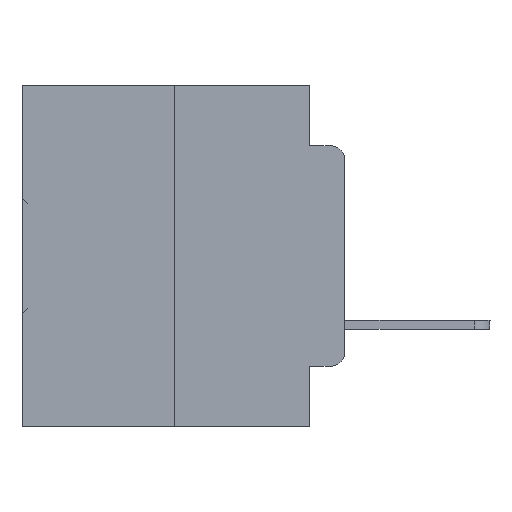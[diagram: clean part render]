
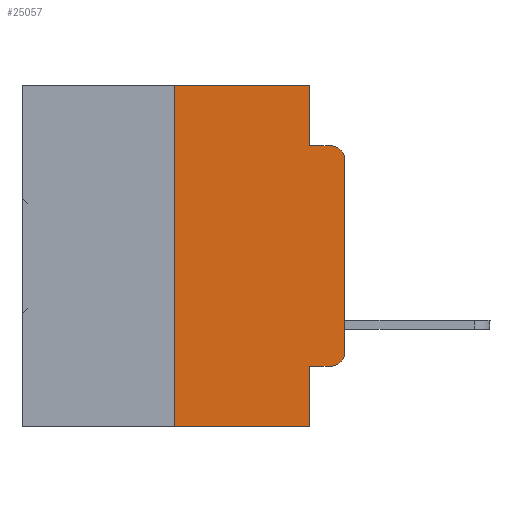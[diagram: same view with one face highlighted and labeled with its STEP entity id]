
A CAD part, left-side view. The second image highlights one B-rep face of the part: STEP entity #25057.
In plain terms, the highlighted planar face has unit normal (-1, 0, 0).
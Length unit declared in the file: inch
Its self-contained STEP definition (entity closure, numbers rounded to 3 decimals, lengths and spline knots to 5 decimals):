
#1318 = CARTESIAN_POINT ( 'NONE',  ( 0., 0.051, 0. ) ) ;
#2047 = LINE ( 'NONE', #31081, #30390 ) ;
#2204 = VECTOR ( 'NONE', #14215, 39.37008 ) ;
#2212 = DIRECTION ( 'NONE',  ( -1., 0., 0. ) ) ;
#2331 = EDGE_CURVE ( 'NONE', #7059, #11870, #3549, .T. ) ;
#2348 = CARTESIAN_POINT ( 'NONE',  ( 0., 0.473, 0. ) ) ;
#2488 = CARTESIAN_POINT ( 'NONE',  ( 0., 0., -0.3915 ) ) ;
#2904 = CARTESIAN_POINT ( 'NONE',  ( 0., 0.25, 0. ) ) ;
#3352 = VECTOR ( 'NONE', #30201, 39.37008 ) ;
#3549 = LINE ( 'NONE', #2904, #31123 ) ;
#3977 = DIRECTION ( 'NONE',  ( 0., 0., -1. ) ) ;
#4874 = DIRECTION ( 'NONE',  ( 0., 0., -1. ) ) ;
#4950 = EDGE_CURVE ( 'NONE', #33336, #5134, #11704, .T. ) ;
#5134 = VERTEX_POINT ( 'NONE', #10693 ) ;
#5249 = CARTESIAN_POINT ( 'NONE',  ( 0., 0.25, -0.5 ) ) ;
#5329 = VERTEX_POINT ( 'NONE', #10025 ) ;
#5924 = VERTEX_POINT ( 'NONE', #24668 ) ;
#5990 = CARTESIAN_POINT ( 'NONE',  ( 0., 0.051, 0. ) ) ;
#6209 = CARTESIAN_POINT ( 'NONE',  ( 0., 0.02, -0.4115 ) ) ;
#7059 = VERTEX_POINT ( 'NONE', #5249 ) ;
#7148 = CARTESIAN_POINT ( 'NONE',  ( 0., 0., 0. ) ) ;
#7413 = VERTEX_POINT ( 'NONE', #17175 ) ;
#7414 = ORIENTED_EDGE ( 'NONE', *, *, #16962, .T. ) ;
#8046 = ORIENTED_EDGE ( 'NONE', *, *, #30200, .T. ) ;
#8646 = ORIENTED_EDGE ( 'NONE', *, *, #21907, .F. ) ;
#9737 = EDGE_CURVE ( 'NONE', #7413, #5329, #22104, .T. ) ;
#9837 = CARTESIAN_POINT ( 'NONE',  ( 0., 0.051, -0.0885 ) ) ;
#9889 = EDGE_CURVE ( 'NONE', #7413, #15257, #2047, .T. ) ;
#10025 = CARTESIAN_POINT ( 'NONE',  ( 0., 0.051, -0.5 ) ) ;
#10128 = VERTEX_POINT ( 'NONE', #18268 ) ;
#10693 = CARTESIAN_POINT ( 'NONE',  ( 0., 0.02, -0.0885 ) ) ;
#11304 = CARTESIAN_POINT ( 'NONE',  ( 0., 0.473, 0. ) ) ;
#11704 = CIRCLE ( 'NONE', #29893, 0.02 ) ;
#11870 = VERTEX_POINT ( 'NONE', #31452 ) ;
#13211 = VECTOR ( 'NONE', #25469, 39.37008 ) ;
#13961 = DIRECTION ( 'NONE',  ( -1., 0., 0. ) ) ;
#14215 = DIRECTION ( 'NONE',  ( 0., 0., -1. ) ) ;
#14391 = ORIENTED_EDGE ( 'NONE', *, *, #32331, .F. ) ;
#15200 = CARTESIAN_POINT ( 'NONE',  ( 0., 0.02, -0.1085 ) ) ;
#15257 = VERTEX_POINT ( 'NONE', #6209 ) ;
#15479 = CARTESIAN_POINT ( 'NONE',  ( 0., 0., -0.1085 ) ) ;
#16403 = LINE ( 'NONE', #9837, #34290 ) ;
#16536 = CARTESIAN_POINT ( 'NONE',  ( 0., 0.02, -0.3915 ) ) ;
#16723 = PLANE ( 'NONE',  #17132 ) ;
#16962 = EDGE_CURVE ( 'NONE', #7059, #5329, #28005, .T. ) ;
#17132 = AXIS2_PLACEMENT_3D ( 'NONE', #11304, #24705, #30069 ) ;
#17175 = CARTESIAN_POINT ( 'NONE',  ( 0., 0.051, -0.4115 ) ) ;
#17361 = LINE ( 'NONE', #2348, #34406 ) ;
#17854 = DIRECTION ( 'NONE',  ( 0., -1., 0. ) ) ;
#17948 = DIRECTION ( 'NONE',  ( 0., -1., 0. ) ) ;
#18268 = CARTESIAN_POINT ( 'NONE',  ( 0., 0.051, 0. ) ) ;
#19103 = ORIENTED_EDGE ( 'NONE', *, *, #2331, .F. ) ;
#19495 = ORIENTED_EDGE ( 'NONE', *, *, #30964, .F. ) ;
#19904 = EDGE_LOOP ( 'NONE', ( #8046, #32866, #8646, #14391, #19495, #19103, #7414, #20446, #33249, #20862 ) ) ;
#20389 = EDGE_CURVE ( 'NONE', #15257, #30312, #26179, .T. ) ;
#20446 = ORIENTED_EDGE ( 'NONE', *, *, #9737, .F. ) ;
#20862 = ORIENTED_EDGE ( 'NONE', *, *, #20389, .T. ) ;
#21623 = DIRECTION ( 'NONE',  ( 0., 0., 1. ) ) ;
#21634 = FACE_OUTER_BOUND ( 'NONE', #19904, .T. ) ;
#21907 = EDGE_CURVE ( 'NONE', #5924, #5134, #16403, .T. ) ;
#22104 = LINE ( 'NONE', #1318, #24568 ) ;
#24568 = VECTOR ( 'NONE', #3977, 39.37008 ) ;
#24668 = CARTESIAN_POINT ( 'NONE',  ( 0., 0.051, -0.0885 ) ) ;
#24705 = DIRECTION ( 'NONE',  ( 1., 0., 0. ) ) ;
#25057 = ADVANCED_FACE ( 'NONE', ( #21634 ), #16723, .F. ) ;
#25469 = DIRECTION ( 'NONE',  ( 0., 0., 1. ) ) ;
#26179 = CIRCLE ( 'NONE', #28481, 0.02 ) ;
#26242 = DIRECTION ( 'NONE',  ( 0., -1., 0. ) ) ;
#28005 = LINE ( 'NONE', #33204, #3352 ) ;
#28481 = AXIS2_PLACEMENT_3D ( 'NONE', #16536, #13961, #32440 ) ;
#29893 = AXIS2_PLACEMENT_3D ( 'NONE', #15200, #2212, #4874 ) ;
#30069 = DIRECTION ( 'NONE',  ( 0., 0., -1. ) ) ;
#30200 = EDGE_CURVE ( 'NONE', #30312, #33336, #33628, .T. ) ;
#30201 = DIRECTION ( 'NONE',  ( 0., -1., 0. ) ) ;
#30312 = VERTEX_POINT ( 'NONE', #2488 ) ;
#30390 = VECTOR ( 'NONE', #17854, 39.37008 ) ;
#30964 = EDGE_CURVE ( 'NONE', #11870, #10128, #17361, .T. ) ;
#31081 = CARTESIAN_POINT ( 'NONE',  ( 0., 0.051, -0.4115 ) ) ;
#31123 = VECTOR ( 'NONE', #21623, 39.37008 ) ;
#31452 = CARTESIAN_POINT ( 'NONE',  ( 0., 0.25, 0. ) ) ;
#32331 = EDGE_CURVE ( 'NONE', #10128, #5924, #32588, .T. ) ;
#32440 = DIRECTION ( 'NONE',  ( 0., 0., -1. ) ) ;
#32588 = LINE ( 'NONE', #5990, #2204 ) ;
#32866 = ORIENTED_EDGE ( 'NONE', *, *, #4950, .T. ) ;
#33204 = CARTESIAN_POINT ( 'NONE',  ( 0., 0.473, -0.5 ) ) ;
#33249 = ORIENTED_EDGE ( 'NONE', *, *, #9889, .T. ) ;
#33336 = VERTEX_POINT ( 'NONE', #15479 ) ;
#33628 = LINE ( 'NONE', #7148, #13211 ) ;
#34290 = VECTOR ( 'NONE', #17948, 39.37008 ) ;
#34406 = VECTOR ( 'NONE', #26242, 39.37008 ) ;
